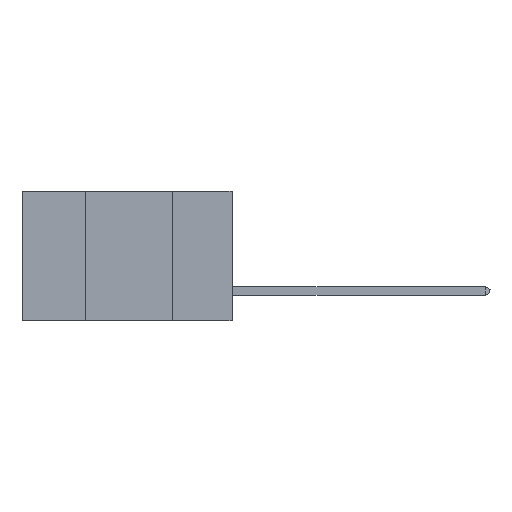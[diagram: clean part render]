
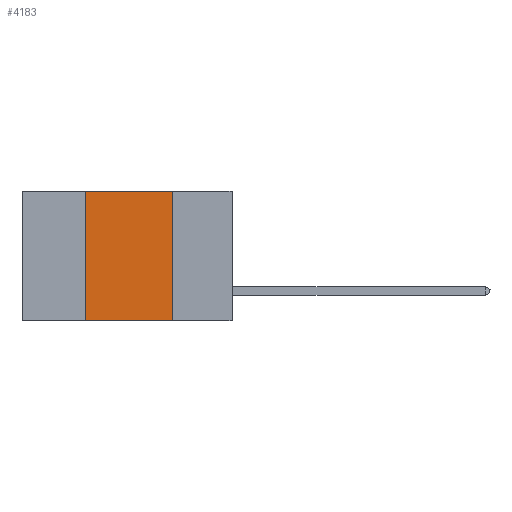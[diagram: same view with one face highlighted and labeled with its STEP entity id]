
A CAD part, left-side view. The second image highlights one B-rep face of the part: STEP entity #4183.
In plain terms, the highlighted planar face has unit normal (-1, 0, 0).
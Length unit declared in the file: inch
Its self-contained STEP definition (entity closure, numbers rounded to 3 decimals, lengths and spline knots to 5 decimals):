
#183 = EDGE_CURVE ( 'NONE', #30539, #14536, #8336, .T. ) ;
#2429 = AXIS2_PLACEMENT_3D ( 'NONE', #7799, #22564, #19112 ) ;
#2537 = LINE ( 'NONE', #24297, #29362 ) ;
#3686 = EDGE_LOOP ( 'NONE', ( #20935, #31833, #14803, #5903 ) ) ;
#4183 = ADVANCED_FACE ( 'NONE', ( #8521 ), #22282, .F. ) ;
#4616 = CARTESIAN_POINT ( 'NONE',  ( 0., 0.17, -0.37 ) ) ;
#5836 = DIRECTION ( 'NONE',  ( 0., -1., 0. ) ) ;
#5903 = ORIENTED_EDGE ( 'NONE', *, *, #25778, .T. ) ;
#6195 = DIRECTION ( 'NONE',  ( 0., 0., -1. ) ) ;
#6477 = CARTESIAN_POINT ( 'NONE',  ( 0., 0.17, 0. ) ) ;
#7289 = VECTOR ( 'NONE', #6195, 39.37008 ) ;
#7799 = CARTESIAN_POINT ( 'NONE',  ( 0., 0.6, 0. ) ) ;
#8238 = DIRECTION ( 'NONE',  ( 0., 0., 1. ) ) ;
#8336 = LINE ( 'NONE', #23804, #21356 ) ;
#8521 = FACE_OUTER_BOUND ( 'NONE', #3686, .T. ) ;
#9198 = VERTEX_POINT ( 'NONE', #6477 ) ;
#9204 = VECTOR ( 'NONE', #5836, 39.37008 ) ;
#14231 = EDGE_CURVE ( 'NONE', #14536, #9198, #27541, .T. ) ;
#14536 = VERTEX_POINT ( 'NONE', #29643 ) ;
#14803 = ORIENTED_EDGE ( 'NONE', *, *, #183, .F. ) ;
#16419 = DIRECTION ( 'NONE',  ( 0., -1., 0. ) ) ;
#18947 = EDGE_CURVE ( 'NONE', #9198, #28383, #25630, .T. ) ;
#19112 = DIRECTION ( 'NONE',  ( 0., 0., -1. ) ) ;
#20935 = ORIENTED_EDGE ( 'NONE', *, *, #18947, .F. ) ;
#21356 = VECTOR ( 'NONE', #8238, 39.37008 ) ;
#21776 = CARTESIAN_POINT ( 'NONE',  ( 0., 0.17, 0. ) ) ;
#22282 = PLANE ( 'NONE',  #2429 ) ;
#22564 = DIRECTION ( 'NONE',  ( 1., 0., 0. ) ) ;
#23804 = CARTESIAN_POINT ( 'NONE',  ( 0., 0.42, 0. ) ) ;
#24112 = CARTESIAN_POINT ( 'NONE',  ( 0., 0.6, 0. ) ) ;
#24297 = CARTESIAN_POINT ( 'NONE',  ( 0., 0.6, -0.37 ) ) ;
#25630 = LINE ( 'NONE', #21776, #7289 ) ;
#25778 = EDGE_CURVE ( 'NONE', #30539, #28383, #2537, .T. ) ;
#27541 = LINE ( 'NONE', #24112, #9204 ) ;
#28383 = VERTEX_POINT ( 'NONE', #4616 ) ;
#29362 = VECTOR ( 'NONE', #16419, 39.37008 ) ;
#29643 = CARTESIAN_POINT ( 'NONE',  ( 0., 0.42, 0. ) ) ;
#30539 = VERTEX_POINT ( 'NONE', #32886 ) ;
#31833 = ORIENTED_EDGE ( 'NONE', *, *, #14231, .F. ) ;
#32886 = CARTESIAN_POINT ( 'NONE',  ( 0., 0.42, -0.37 ) ) ;
